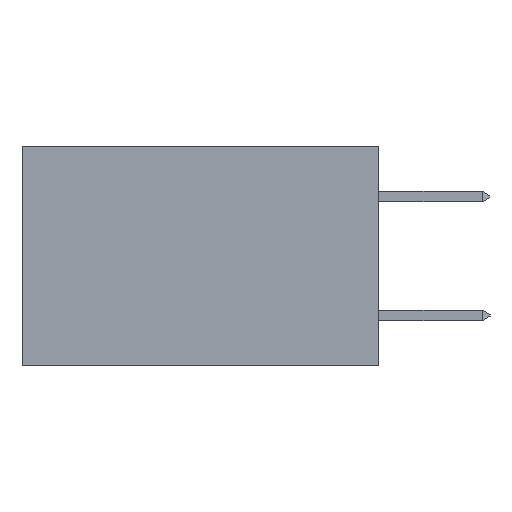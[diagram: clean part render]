
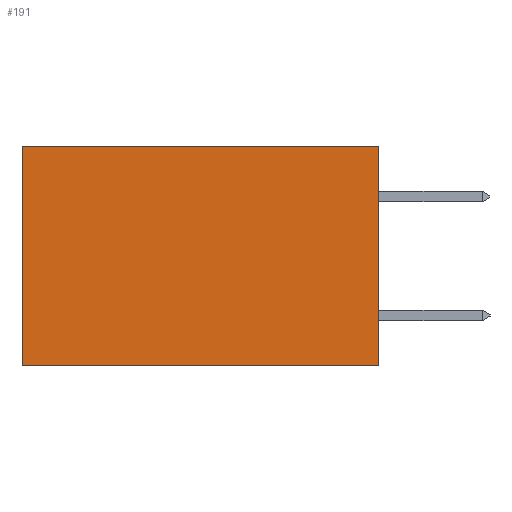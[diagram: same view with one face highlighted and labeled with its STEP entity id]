
A CAD part, left-side view. The second image highlights one B-rep face of the part: STEP entity #191.
In plain terms, the highlighted planar face has unit normal (-1, 0, 0).
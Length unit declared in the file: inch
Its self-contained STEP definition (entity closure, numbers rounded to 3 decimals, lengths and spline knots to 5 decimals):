
#191 = ADVANCED_FACE ( 'NONE', ( #6792 ), #9370, .F. ) ;
#402 = CARTESIAN_POINT ( 'NONE',  ( 0.2615, 0.6, 0. ) ) ;
#2031 = EDGE_CURVE ( 'NONE', #3884, #14581, #20568, .T. ) ;
#2081 = CARTESIAN_POINT ( 'NONE',  ( 0.2615, 0., 0. ) ) ;
#2897 = EDGE_LOOP ( 'NONE', ( #5012, #13196, #16053, #22173 ) ) ;
#3346 = LINE ( 'NONE', #18553, #12739 ) ;
#3884 = VERTEX_POINT ( 'NONE', #2081 ) ;
#4521 = EDGE_CURVE ( 'NONE', #3884, #9204, #3346, .T. ) ;
#5012 = ORIENTED_EDGE ( 'NONE', *, *, #12911, .T. ) ;
#6131 = CARTESIAN_POINT ( 'NONE',  ( 0.2615, 0., -0.37 ) ) ;
#6150 = LINE ( 'NONE', #12547, #15586 ) ;
#6656 = EDGE_CURVE ( 'NONE', #9204, #10340, #6150, .T. ) ;
#6792 = FACE_OUTER_BOUND ( 'NONE', #2897, .T. ) ;
#7065 = DIRECTION ( 'NONE',  ( 0., 0., -1. ) ) ;
#7215 = DIRECTION ( 'NONE',  ( 1., 0., 0. ) ) ;
#7957 = CARTESIAN_POINT ( 'NONE',  ( 0.2615, 0., -0.37 ) ) ;
#9204 = VERTEX_POINT ( 'NONE', #6131 ) ;
#9360 = DIRECTION ( 'NONE',  ( 0., 0., -1. ) ) ;
#9370 = PLANE ( 'NONE',  #19390 ) ;
#10340 = VERTEX_POINT ( 'NONE', #10945 ) ;
#10945 = CARTESIAN_POINT ( 'NONE',  ( 0.2615, 0.6, -0.37 ) ) ;
#11140 = VECTOR ( 'NONE', #12968, 39.37008 ) ;
#11710 = CARTESIAN_POINT ( 'NONE',  ( 0.2615, 0., 0. ) ) ;
#12547 = CARTESIAN_POINT ( 'NONE',  ( 0.2615, 0., -0.37 ) ) ;
#12646 = DIRECTION ( 'NONE',  ( 0., 1., 0. ) ) ;
#12739 = VECTOR ( 'NONE', #9360, 39.37008 ) ;
#12911 = EDGE_CURVE ( 'NONE', #14581, #10340, #19783, .T. ) ;
#12968 = DIRECTION ( 'NONE',  ( 0., 1., 0. ) ) ;
#13196 = ORIENTED_EDGE ( 'NONE', *, *, #6656, .F. ) ;
#13588 = DIRECTION ( 'NONE',  ( 0., 0., -1. ) ) ;
#14581 = VERTEX_POINT ( 'NONE', #402 ) ;
#14786 = VECTOR ( 'NONE', #13588, 39.37008 ) ;
#15586 = VECTOR ( 'NONE', #12646, 39.37008 ) ;
#16053 = ORIENTED_EDGE ( 'NONE', *, *, #4521, .F. ) ;
#18553 = CARTESIAN_POINT ( 'NONE',  ( 0.2615, 0., -0.37 ) ) ;
#19390 = AXIS2_PLACEMENT_3D ( 'NONE', #7957, #7215, #7065 ) ;
#19783 = LINE ( 'NONE', #22980, #14786 ) ;
#20568 = LINE ( 'NONE', #11710, #11140 ) ;
#22173 = ORIENTED_EDGE ( 'NONE', *, *, #2031, .T. ) ;
#22980 = CARTESIAN_POINT ( 'NONE',  ( 0.2615, 0.6, -0.37 ) ) ;
